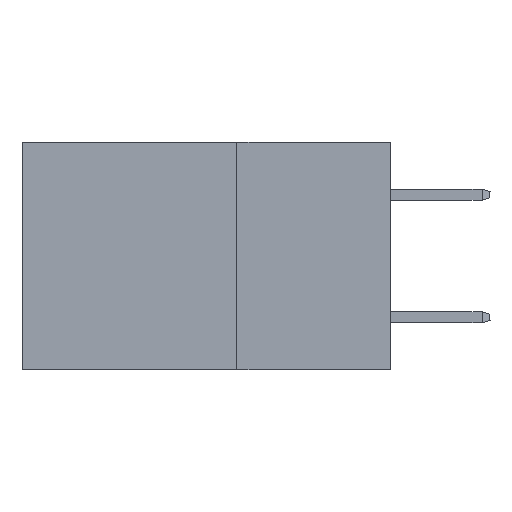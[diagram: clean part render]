
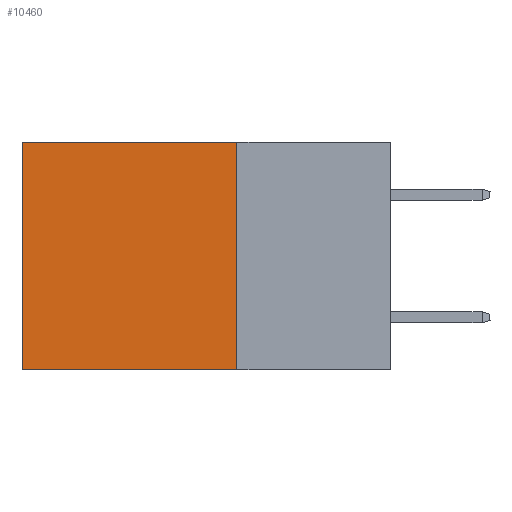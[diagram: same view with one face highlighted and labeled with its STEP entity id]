
A CAD part, left-side view. The second image highlights one B-rep face of the part: STEP entity #10460.
In plain terms, the highlighted planar face has unit normal (-1, 0, 0).
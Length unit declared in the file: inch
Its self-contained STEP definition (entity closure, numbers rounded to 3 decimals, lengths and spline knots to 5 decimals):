
#663 = EDGE_CURVE ( 'NONE', #15827, #1183, #18850, .T. ) ;
#950 = VECTOR ( 'NONE', #22155, 39.37008 ) ;
#1183 = VERTEX_POINT ( 'NONE', #5201 ) ;
#2710 = LINE ( 'NONE', #13663, #6648 ) ;
#3269 = VERTEX_POINT ( 'NONE', #26317 ) ;
#3342 = CARTESIAN_POINT ( 'NONE',  ( 0.2875, 0.25, 0. ) ) ;
#3355 = DIRECTION ( 'NONE',  ( 0., 1., 0. ) ) ;
#3943 = EDGE_LOOP ( 'NONE', ( #22464, #23125, #22792, #25078 ) ) ;
#5201 = CARTESIAN_POINT ( 'NONE',  ( 0.2875, 0.25, -0.37 ) ) ;
#6648 = VECTOR ( 'NONE', #3355, 39.37008 ) ;
#6700 = AXIS2_PLACEMENT_3D ( 'NONE', #14304, #18525, #20618 ) ;
#7131 = EDGE_CURVE ( 'NONE', #15827, #3269, #12133, .T. ) ;
#7574 = CARTESIAN_POINT ( 'NONE',  ( 0.2875, 0.6, -0.37 ) ) ;
#9163 = LINE ( 'NONE', #10798, #19660 ) ;
#10460 = ADVANCED_FACE ( 'NONE', ( #17174 ), #24687, .F. ) ;
#10798 = CARTESIAN_POINT ( 'NONE',  ( 0.2875, 0.6, 0. ) ) ;
#11600 = DIRECTION ( 'NONE',  ( 0., 0., -1. ) ) ;
#12133 = LINE ( 'NONE', #3342, #950 ) ;
#12229 = CARTESIAN_POINT ( 'NONE',  ( 0.2875, 0.25, 0. ) ) ;
#13257 = EDGE_CURVE ( 'NONE', #3269, #13932, #9163, .T. ) ;
#13663 = CARTESIAN_POINT ( 'NONE',  ( 0.2875, 0.25, -0.37 ) ) ;
#13932 = VERTEX_POINT ( 'NONE', #7574 ) ;
#14304 = CARTESIAN_POINT ( 'NONE',  ( 0.2875, 0.25, 0. ) ) ;
#15007 = DIRECTION ( 'NONE',  ( 0., 0., -1. ) ) ;
#15827 = VERTEX_POINT ( 'NONE', #12229 ) ;
#17174 = FACE_OUTER_BOUND ( 'NONE', #3943, .T. ) ;
#17618 = EDGE_CURVE ( 'NONE', #1183, #13932, #2710, .T. ) ;
#18525 = DIRECTION ( 'NONE',  ( 1., 0., 0. ) ) ;
#18850 = LINE ( 'NONE', #19701, #24045 ) ;
#19660 = VECTOR ( 'NONE', #15007, 39.37008 ) ;
#19701 = CARTESIAN_POINT ( 'NONE',  ( 0.2875, 0.25, 0. ) ) ;
#20618 = DIRECTION ( 'NONE',  ( 0., 0., -1. ) ) ;
#22155 = DIRECTION ( 'NONE',  ( 0., 1., 0. ) ) ;
#22464 = ORIENTED_EDGE ( 'NONE', *, *, #13257, .T. ) ;
#22792 = ORIENTED_EDGE ( 'NONE', *, *, #663, .F. ) ;
#23125 = ORIENTED_EDGE ( 'NONE', *, *, #17618, .F. ) ;
#24045 = VECTOR ( 'NONE', #11600, 39.37008 ) ;
#24687 = PLANE ( 'NONE',  #6700 ) ;
#25078 = ORIENTED_EDGE ( 'NONE', *, *, #7131, .T. ) ;
#26317 = CARTESIAN_POINT ( 'NONE',  ( 0.2875, 0.6, 0. ) ) ;
